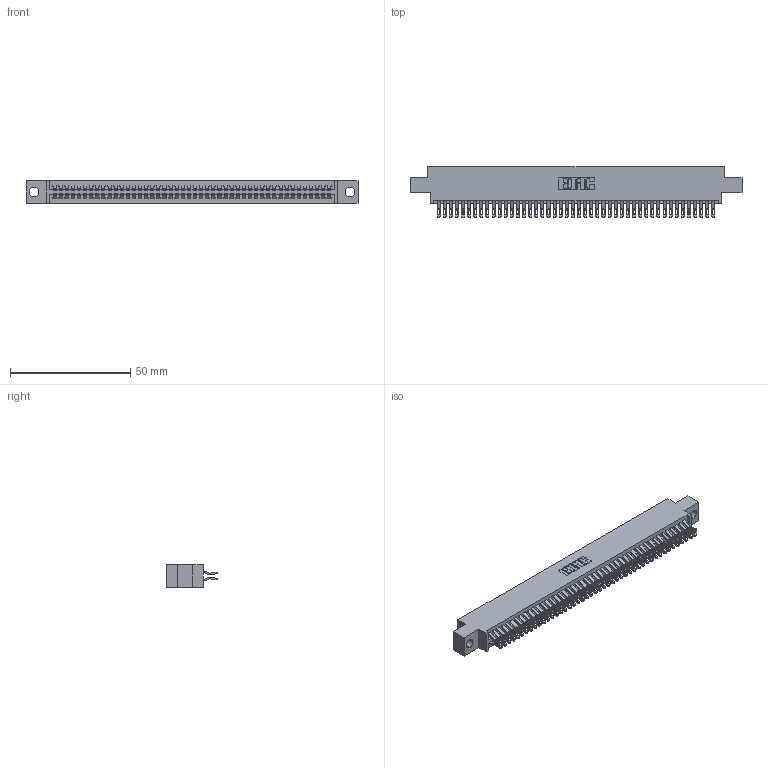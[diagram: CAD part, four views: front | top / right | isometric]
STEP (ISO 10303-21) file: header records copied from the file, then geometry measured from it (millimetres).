
FILE_DESCRIPTION (( 'STEP AP203' ), '1' );
FILE_NAME ('395-092-555-804.STEP', '2018-11-29T08:53:34', ( '' ), ( '' ), 'SwSTEP 2.0', 'SolidWorks 2016', '' );
FILE_SCHEMA (( 'CONFIG_CONTROL_DESIGN' ));
Length unit declared in the file: inch
Products named in the file (3): 345-292-001_555 Tail; 345 Part_0.170 Offset - 0.156 Dia-TH; 395-092-555-804
Assembly tree (93 placements, depth 2):
  395-092-555-804
    345 Part_0.170 Offset - 0.156 Dia-TH
    345-292-001_555 Tail  x92
Bounding box: 138.05 x 21.13 x 9.4 mm (x, y, z)
Volume: 13513 mm3; surface area: 20938.7 mm2
Topology: 93 solids, 93 shells, 5282 faces, 16637 edges, 11090 vertices
Faces by surface type: plane 2936, cylinder 2346
Entity records: 36015 total; most frequent: CARTESIAN_POINT 6070, ORIENTED_EDGE 5974, DIRECTION 5315, EDGE_CURVE 2987, LINE 2651, VECTOR 2651, VERTEX_POINT 1990, AXIS2_PLACEMENT_3D 1332
